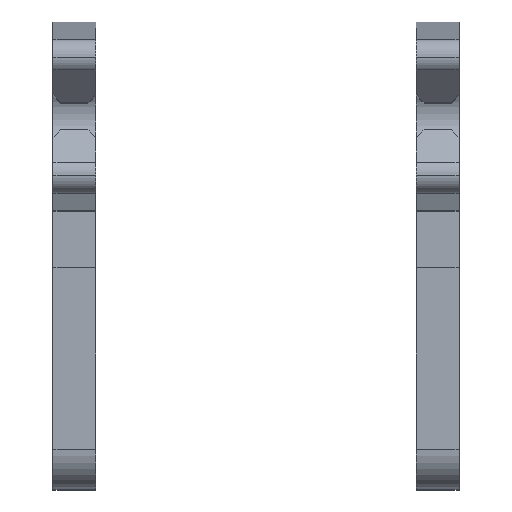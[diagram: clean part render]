
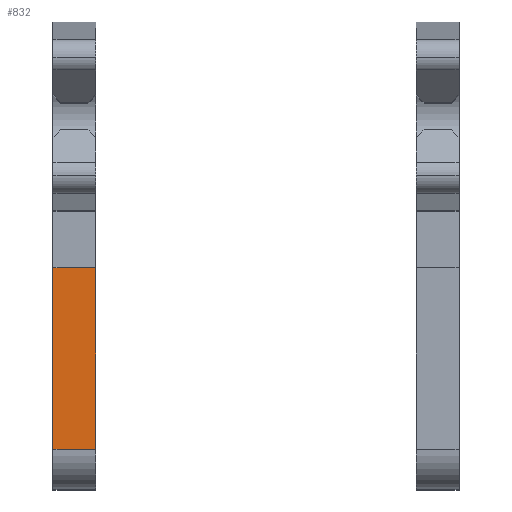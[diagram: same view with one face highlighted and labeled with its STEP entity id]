
A CAD part, top view. The second image highlights one B-rep face of the part: STEP entity #832.
In plain terms, the highlighted planar face has unit normal (0, 0, 1).
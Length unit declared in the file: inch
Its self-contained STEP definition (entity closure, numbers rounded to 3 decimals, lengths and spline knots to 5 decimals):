
#55 = LINE ( 'NONE', #1006, #294 ) ;
#85 = DIRECTION ( 'NONE',  ( -1., 0., 0. ) ) ;
#133 = FACE_OUTER_BOUND ( 'NONE', #416, .T. ) ;
#150 = VECTOR ( 'NONE', #199, 39.37008 ) ;
#172 = CARTESIAN_POINT ( 'NONE',  ( 0.0118, -0.183, -0.058 ) ) ;
#196 = VERTEX_POINT ( 'NONE', #172 ) ;
#199 = DIRECTION ( 'NONE',  ( 0., -1., 0. ) ) ;
#269 = CARTESIAN_POINT ( 'NONE',  ( 0.0118, -0.083, -0.058 ) ) ;
#270 = VECTOR ( 'NONE', #353, 39.37008 ) ;
#283 = DIRECTION ( 'NONE',  ( -1., 0., 0. ) ) ;
#294 = VECTOR ( 'NONE', #85, 39.37008 ) ;
#303 = ORIENTED_EDGE ( 'NONE', *, *, #556, .T. ) ;
#353 = DIRECTION ( 'NONE',  ( 0., -1., 0. ) ) ;
#407 = ORIENTED_EDGE ( 'NONE', *, *, #562, .T. ) ;
#416 = EDGE_LOOP ( 'NONE', ( #407, #695, #1092, #303 ) ) ;
#446 = EDGE_CURVE ( 'NONE', #196, #1123, #55, .T. ) ;
#459 = DIRECTION ( 'NONE',  ( 0., 0., -1. ) ) ;
#476 = VERTEX_POINT ( 'NONE', #1097 ) ;
#519 = CARTESIAN_POINT ( 'NONE',  ( 0.0118, -0.083, -0.058 ) ) ;
#556 = EDGE_CURVE ( 'NONE', #578, #476, #958, .T. ) ;
#562 = EDGE_CURVE ( 'NONE', #476, #1123, #1161, .T. ) ;
#578 = VERTEX_POINT ( 'NONE', #269 ) ;
#648 = CARTESIAN_POINT ( 'NONE',  ( 0.0118, -0.183, -0.058 ) ) ;
#695 = ORIENTED_EDGE ( 'NONE', *, *, #446, .F. ) ;
#716 = VECTOR ( 'NONE', #784, 39.37008 ) ;
#784 = DIRECTION ( 'NONE',  ( -1., 0., 0. ) ) ;
#812 = AXIS2_PLACEMENT_3D ( 'NONE', #1124, #459, #283 ) ;
#819 = EDGE_CURVE ( 'NONE', #578, #196, #1045, .T. ) ;
#832 = ADVANCED_FACE ( 'NONE', ( #133 ), #916, .F. ) ;
#916 = PLANE ( 'NONE',  #812 ) ;
#958 = LINE ( 'NONE', #519, #716 ) ;
#977 = CARTESIAN_POINT ( 'NONE',  ( -0.0118, -0.183, -0.058 ) ) ;
#994 = CARTESIAN_POINT ( 'NONE',  ( -0.0118, -0.183, -0.058 ) ) ;
#1006 = CARTESIAN_POINT ( 'NONE',  ( 0.0118, -0.183, -0.058 ) ) ;
#1045 = LINE ( 'NONE', #648, #150 ) ;
#1092 = ORIENTED_EDGE ( 'NONE', *, *, #819, .F. ) ;
#1097 = CARTESIAN_POINT ( 'NONE',  ( -0.0118, -0.083, -0.058 ) ) ;
#1123 = VERTEX_POINT ( 'NONE', #977 ) ;
#1124 = CARTESIAN_POINT ( 'NONE',  ( 0.0118, -0.183, -0.058 ) ) ;
#1161 = LINE ( 'NONE', #994, #270 ) ;
